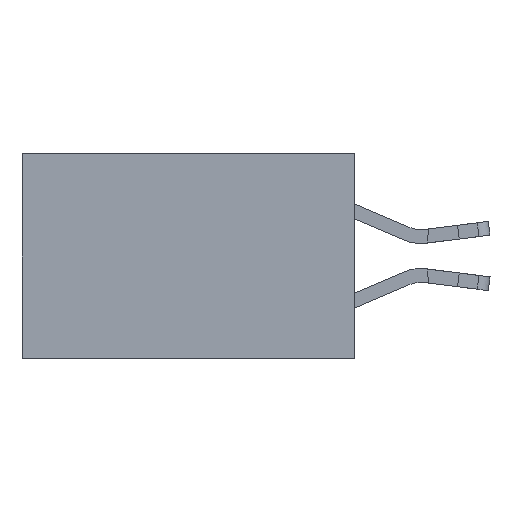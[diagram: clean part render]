
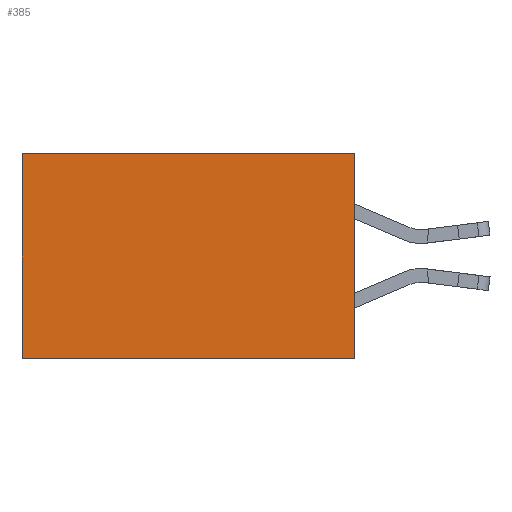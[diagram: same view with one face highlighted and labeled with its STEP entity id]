
A CAD part, left-side view. The second image highlights one B-rep face of the part: STEP entity #385.
In plain terms, the highlighted planar face has unit normal (-1, 0, 0).
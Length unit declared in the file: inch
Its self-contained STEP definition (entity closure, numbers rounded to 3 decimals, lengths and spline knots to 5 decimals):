
#113 = VERTEX_POINT ( 'NONE', #1884 ) ;
#385 = ADVANCED_FACE ( 'NONE', ( #7168 ), #16981, .F. ) ;
#1028 = EDGE_LOOP ( 'NONE', ( #14848, #2254, #8874, #5265 ) ) ;
#1884 = CARTESIAN_POINT ( 'NONE',  ( 0.2615, 0., 0. ) ) ;
#2254 = ORIENTED_EDGE ( 'NONE', *, *, #10625, .F. ) ;
#2951 = CARTESIAN_POINT ( 'NONE',  ( 0.2615, 0., -0.37 ) ) ;
#3704 = LINE ( 'NONE', #10587, #15245 ) ;
#4197 = EDGE_CURVE ( 'NONE', #113, #10693, #3704, .T. ) ;
#5265 = ORIENTED_EDGE ( 'NONE', *, *, #4197, .T. ) ;
#5561 = CARTESIAN_POINT ( 'NONE',  ( 0.2615, 0.6, -0.37 ) ) ;
#6391 = EDGE_CURVE ( 'NONE', #113, #9579, #9788, .T. ) ;
#6700 = CARTESIAN_POINT ( 'NONE',  ( 0.2615, 0.6, -0.37 ) ) ;
#6878 = CARTESIAN_POINT ( 'NONE',  ( 0.2615, 0., -0.37 ) ) ;
#7168 = FACE_OUTER_BOUND ( 'NONE', #1028, .T. ) ;
#7896 = DIRECTION ( 'NONE',  ( 0., 0., -1. ) ) ;
#8409 = AXIS2_PLACEMENT_3D ( 'NONE', #6878, #10804, #7896 ) ;
#8465 = VERTEX_POINT ( 'NONE', #6700 ) ;
#8874 = ORIENTED_EDGE ( 'NONE', *, *, #6391, .F. ) ;
#8956 = LINE ( 'NONE', #5561, #9440 ) ;
#9388 = EDGE_CURVE ( 'NONE', #10693, #8465, #8956, .T. ) ;
#9440 = VECTOR ( 'NONE', #16091, 39.37008 ) ;
#9579 = VERTEX_POINT ( 'NONE', #2951 ) ;
#9788 = LINE ( 'NONE', #11208, #13327 ) ;
#10331 = LINE ( 'NONE', #17386, #17778 ) ;
#10459 = DIRECTION ( 'NONE',  ( 0., 1., 0. ) ) ;
#10587 = CARTESIAN_POINT ( 'NONE',  ( 0.2615, 0., 0. ) ) ;
#10625 = EDGE_CURVE ( 'NONE', #9579, #8465, #10331, .T. ) ;
#10693 = VERTEX_POINT ( 'NONE', #17514 ) ;
#10804 = DIRECTION ( 'NONE',  ( 1., 0., 0. ) ) ;
#11208 = CARTESIAN_POINT ( 'NONE',  ( 0.2615, 0., -0.37 ) ) ;
#13327 = VECTOR ( 'NONE', #14205, 39.37008 ) ;
#14205 = DIRECTION ( 'NONE',  ( 0., 0., -1. ) ) ;
#14848 = ORIENTED_EDGE ( 'NONE', *, *, #9388, .T. ) ;
#15245 = VECTOR ( 'NONE', #10459, 39.37008 ) ;
#16091 = DIRECTION ( 'NONE',  ( 0., 0., -1. ) ) ;
#16981 = PLANE ( 'NONE',  #8409 ) ;
#17386 = CARTESIAN_POINT ( 'NONE',  ( 0.2615, 0., -0.37 ) ) ;
#17514 = CARTESIAN_POINT ( 'NONE',  ( 0.2615, 0.6, 0. ) ) ;
#17778 = VECTOR ( 'NONE', #18864, 39.37008 ) ;
#18864 = DIRECTION ( 'NONE',  ( 0., 1., 0. ) ) ;
